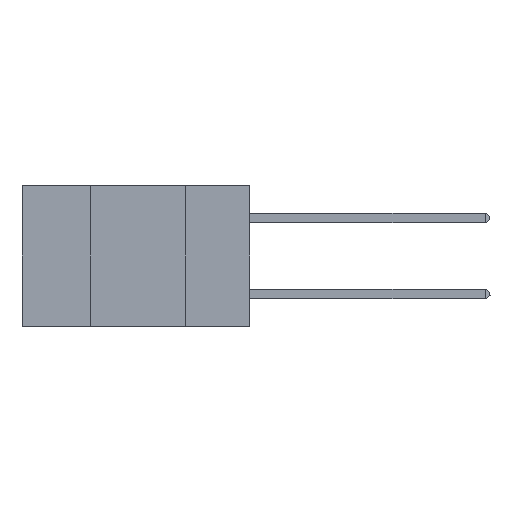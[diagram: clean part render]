
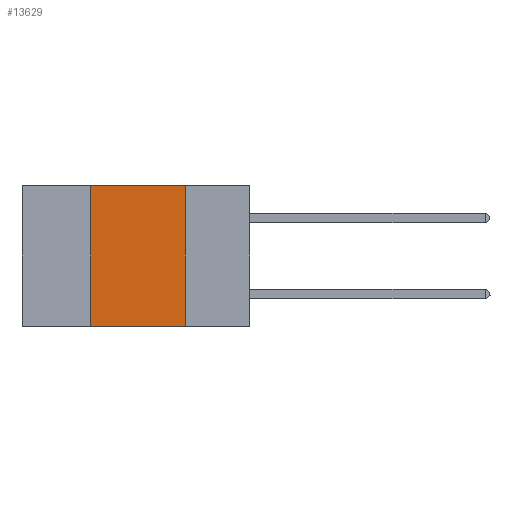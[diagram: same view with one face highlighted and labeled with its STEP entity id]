
A CAD part, left-side view. The second image highlights one B-rep face of the part: STEP entity #13629.
In plain terms, the highlighted planar face has unit normal (-1, 0, 0).
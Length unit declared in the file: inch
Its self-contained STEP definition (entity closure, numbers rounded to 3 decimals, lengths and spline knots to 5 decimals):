
#140 = EDGE_CURVE ( 'NONE', #1089, #2451, #18613, .T. ) ;
#1089 = VERTEX_POINT ( 'NONE', #7045 ) ;
#2451 = VERTEX_POINT ( 'NONE', #13697 ) ;
#2460 = ORIENTED_EDGE ( 'NONE', *, *, #10378, .F. ) ;
#3800 = LINE ( 'NONE', #23068, #11633 ) ;
#6066 = CARTESIAN_POINT ( 'NONE',  ( 0., 0.42, 0. ) ) ;
#7045 = CARTESIAN_POINT ( 'NONE',  ( 0., 0.42, -0.37 ) ) ;
#8694 = ORIENTED_EDGE ( 'NONE', *, *, #25114, .F. ) ;
#9453 = DIRECTION ( 'NONE',  ( 0., 0., -1. ) ) ;
#9542 = VECTOR ( 'NONE', #26233, 39.37008 ) ;
#10246 = CARTESIAN_POINT ( 'NONE',  ( 0., 0.42, 0. ) ) ;
#10378 = EDGE_CURVE ( 'NONE', #17233, #2451, #3800, .T. ) ;
#11633 = VECTOR ( 'NONE', #24242, 39.37008 ) ;
#13629 = ADVANCED_FACE ( 'NONE', ( #14638 ), #19184, .F. ) ;
#13697 = CARTESIAN_POINT ( 'NONE',  ( 0., 0.17, -0.37 ) ) ;
#14638 = FACE_OUTER_BOUND ( 'NONE', #16309, .T. ) ;
#15349 = AXIS2_PLACEMENT_3D ( 'NONE', #29073, #24317, #9453 ) ;
#15828 = DIRECTION ( 'NONE',  ( 0., 0., 1. ) ) ;
#16309 = EDGE_LOOP ( 'NONE', ( #2460, #17431, #8694, #18103 ) ) ;
#17233 = VERTEX_POINT ( 'NONE', #22605 ) ;
#17431 = ORIENTED_EDGE ( 'NONE', *, *, #18297, .F. ) ;
#18103 = ORIENTED_EDGE ( 'NONE', *, *, #140, .T. ) ;
#18297 = EDGE_CURVE ( 'NONE', #24340, #17233, #29948, .T. ) ;
#18613 = LINE ( 'NONE', #30049, #24897 ) ;
#19133 = LINE ( 'NONE', #10246, #30884 ) ;
#19184 = PLANE ( 'NONE',  #15349 ) ;
#20055 = DIRECTION ( 'NONE',  ( 0., -1., 0. ) ) ;
#20659 = CARTESIAN_POINT ( 'NONE',  ( 0., 0.6, 0. ) ) ;
#22605 = CARTESIAN_POINT ( 'NONE',  ( 0., 0.17, 0. ) ) ;
#23068 = CARTESIAN_POINT ( 'NONE',  ( 0., 0.17, 0. ) ) ;
#24242 = DIRECTION ( 'NONE',  ( 0., 0., -1. ) ) ;
#24317 = DIRECTION ( 'NONE',  ( 1., 0., 0. ) ) ;
#24340 = VERTEX_POINT ( 'NONE', #6066 ) ;
#24897 = VECTOR ( 'NONE', #20055, 39.37008 ) ;
#25114 = EDGE_CURVE ( 'NONE', #1089, #24340, #19133, .T. ) ;
#26233 = DIRECTION ( 'NONE',  ( 0., -1., 0. ) ) ;
#29073 = CARTESIAN_POINT ( 'NONE',  ( 0., 0.6, 0. ) ) ;
#29948 = LINE ( 'NONE', #20659, #9542 ) ;
#30049 = CARTESIAN_POINT ( 'NONE',  ( 0., 0.6, -0.37 ) ) ;
#30884 = VECTOR ( 'NONE', #15828, 39.37008 ) ;
